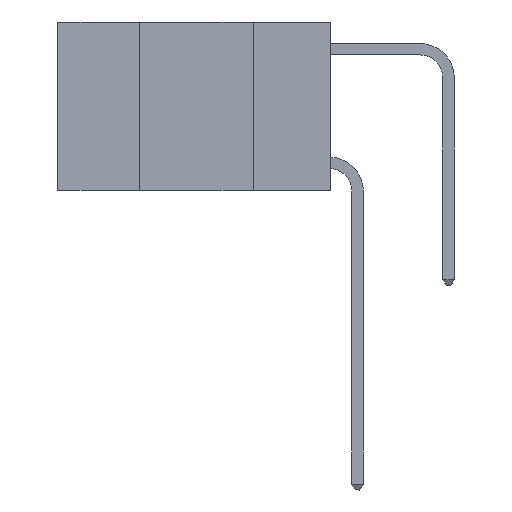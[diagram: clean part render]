
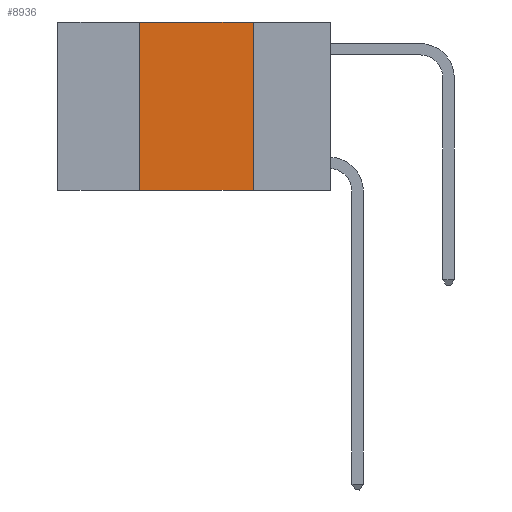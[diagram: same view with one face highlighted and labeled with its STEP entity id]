
A CAD part, left-side view. The second image highlights one B-rep face of the part: STEP entity #8936.
In plain terms, the highlighted planar face has unit normal (-1, 0, 0).
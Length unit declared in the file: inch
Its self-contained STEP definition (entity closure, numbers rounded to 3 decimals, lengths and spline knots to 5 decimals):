
#62 = CARTESIAN_POINT ( 'NONE',  ( 0., 0.6, 0. ) ) ;
#775 = VECTOR ( 'NONE', #4509, 39.37008 ) ;
#1163 = EDGE_CURVE ( 'NONE', #2990, #8326, #12572, .T. ) ;
#1736 = LINE ( 'NONE', #9094, #775 ) ;
#2413 = CARTESIAN_POINT ( 'NONE',  ( 0., 0.17, -0.37 ) ) ;
#2792 = VECTOR ( 'NONE', #3388, 39.37008 ) ;
#2990 = VERTEX_POINT ( 'NONE', #4853 ) ;
#3388 = DIRECTION ( 'NONE',  ( 0., 0., -1. ) ) ;
#3416 = VERTEX_POINT ( 'NONE', #2413 ) ;
#3871 = DIRECTION ( 'NONE',  ( 0., -1., 0. ) ) ;
#3943 = FACE_OUTER_BOUND ( 'NONE', #13042, .T. ) ;
#4509 = DIRECTION ( 'NONE',  ( 0., 0., 1. ) ) ;
#4510 = ORIENTED_EDGE ( 'NONE', *, *, #5999, .F. ) ;
#4607 = CARTESIAN_POINT ( 'NONE',  ( 0., 0.17, 0. ) ) ;
#4716 = ORIENTED_EDGE ( 'NONE', *, *, #5697, .F. ) ;
#4853 = CARTESIAN_POINT ( 'NONE',  ( 0., 0.42, 0. ) ) ;
#5006 = DIRECTION ( 'NONE',  ( 0., 0., -1. ) ) ;
#5337 = DIRECTION ( 'NONE',  ( 1., 0., 0. ) ) ;
#5697 = EDGE_CURVE ( 'NONE', #8326, #3416, #15585, .T. ) ;
#5999 = EDGE_CURVE ( 'NONE', #12684, #2990, #1736, .T. ) ;
#6407 = CARTESIAN_POINT ( 'NONE',  ( 0., 0.42, -0.37 ) ) ;
#7106 = CARTESIAN_POINT ( 'NONE',  ( 0., 0.17, 0. ) ) ;
#7952 = CARTESIAN_POINT ( 'NONE',  ( 0., 0.6, 0. ) ) ;
#8326 = VERTEX_POINT ( 'NONE', #7106 ) ;
#8348 = VECTOR ( 'NONE', #11537, 39.37008 ) ;
#8426 = AXIS2_PLACEMENT_3D ( 'NONE', #62, #5337, #5006 ) ;
#8866 = PLANE ( 'NONE',  #8426 ) ;
#8936 = ADVANCED_FACE ( 'NONE', ( #3943 ), #8866, .F. ) ;
#9094 = CARTESIAN_POINT ( 'NONE',  ( 0., 0.42, 0. ) ) ;
#10511 = ORIENTED_EDGE ( 'NONE', *, *, #1163, .F. ) ;
#11268 = LINE ( 'NONE', #14892, #14146 ) ;
#11537 = DIRECTION ( 'NONE',  ( 0., -1., 0. ) ) ;
#12572 = LINE ( 'NONE', #7952, #8348 ) ;
#12684 = VERTEX_POINT ( 'NONE', #6407 ) ;
#12880 = ORIENTED_EDGE ( 'NONE', *, *, #15812, .T. ) ;
#13042 = EDGE_LOOP ( 'NONE', ( #4716, #10511, #4510, #12880 ) ) ;
#14146 = VECTOR ( 'NONE', #3871, 39.37008 ) ;
#14892 = CARTESIAN_POINT ( 'NONE',  ( 0., 0.6, -0.37 ) ) ;
#15585 = LINE ( 'NONE', #4607, #2792 ) ;
#15812 = EDGE_CURVE ( 'NONE', #12684, #3416, #11268, .T. ) ;
